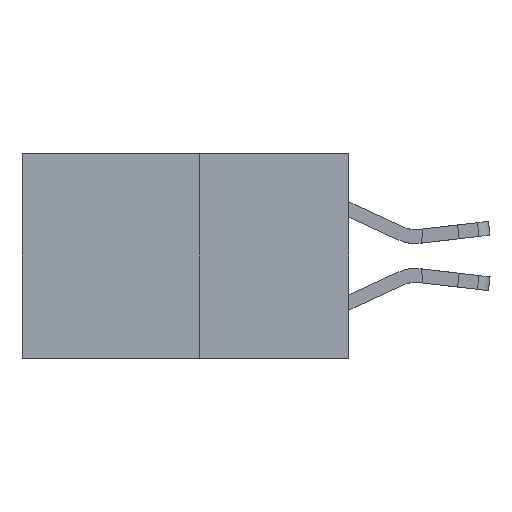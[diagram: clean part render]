
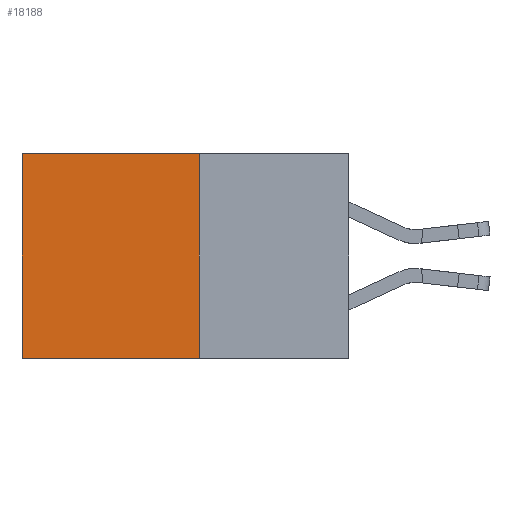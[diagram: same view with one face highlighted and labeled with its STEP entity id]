
A CAD part, left-side view. The second image highlights one B-rep face of the part: STEP entity #18188.
In plain terms, the highlighted planar face has unit normal (-1, 0, 0).
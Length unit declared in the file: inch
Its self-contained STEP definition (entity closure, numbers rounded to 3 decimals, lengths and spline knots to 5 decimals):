
#17 = VERTEX_POINT ( 'NONE', #15358 ) ;
#2304 = LINE ( 'NONE', #13840, #17884 ) ;
#2320 = CARTESIAN_POINT ( 'NONE',  ( 0.277, 0.59, -0.37 ) ) ;
#2510 = LINE ( 'NONE', #18720, #18080 ) ;
#2640 = CARTESIAN_POINT ( 'NONE',  ( 0.277, 0.27, -0.37 ) ) ;
#3442 = FACE_OUTER_BOUND ( 'NONE', #15813, .T. ) ;
#4179 = DIRECTION ( 'NONE',  ( 0., 0., -1. ) ) ;
#4262 = LINE ( 'NONE', #4757, #11395 ) ;
#4757 = CARTESIAN_POINT ( 'NONE',  ( 0.277, 0.27, -0.37 ) ) ;
#4841 = DIRECTION ( 'NONE',  ( 0., 1., 0. ) ) ;
#4848 = CARTESIAN_POINT ( 'NONE',  ( 0.277, 0.27, -0.37 ) ) ;
#5028 = EDGE_CURVE ( 'NONE', #17586, #14754, #2510, .T. ) ;
#5360 = CARTESIAN_POINT ( 'NONE',  ( 0.277, 0.27, 0. ) ) ;
#5529 = DIRECTION ( 'NONE',  ( 0., 1., 0. ) ) ;
#8305 = AXIS2_PLACEMENT_3D ( 'NONE', #2640, #13247, #4179 ) ;
#8691 = ORIENTED_EDGE ( 'NONE', *, *, #16693, .T. ) ;
#9034 = EDGE_CURVE ( 'NONE', #17586, #17, #17234, .T. ) ;
#9090 = EDGE_CURVE ( 'NONE', #14754, #9318, #4262, .T. ) ;
#9318 = VERTEX_POINT ( 'NONE', #2320 ) ;
#9626 = ORIENTED_EDGE ( 'NONE', *, *, #9090, .F. ) ;
#10334 = ORIENTED_EDGE ( 'NONE', *, *, #5028, .F. ) ;
#11395 = VECTOR ( 'NONE', #4841, 39.37008 ) ;
#11746 = PLANE ( 'NONE',  #8305 ) ;
#12327 = VECTOR ( 'NONE', #5529, 39.37008 ) ;
#12668 = CARTESIAN_POINT ( 'NONE',  ( 0.277, 0.27, 0. ) ) ;
#12875 = ORIENTED_EDGE ( 'NONE', *, *, #9034, .T. ) ;
#13247 = DIRECTION ( 'NONE',  ( 1., 0., 0. ) ) ;
#13840 = CARTESIAN_POINT ( 'NONE',  ( 0.277, 0.59, -0.37 ) ) ;
#14754 = VERTEX_POINT ( 'NONE', #4848 ) ;
#15352 = DIRECTION ( 'NONE',  ( 0., 0., -1. ) ) ;
#15358 = CARTESIAN_POINT ( 'NONE',  ( 0.277, 0.59, 0. ) ) ;
#15813 = EDGE_LOOP ( 'NONE', ( #8691, #9626, #10334, #12875 ) ) ;
#16693 = EDGE_CURVE ( 'NONE', #17, #9318, #2304, .T. ) ;
#17234 = LINE ( 'NONE', #5360, #12327 ) ;
#17586 = VERTEX_POINT ( 'NONE', #12668 ) ;
#17884 = VECTOR ( 'NONE', #15352, 39.37008 ) ;
#18080 = VECTOR ( 'NONE', #18573, 39.37008 ) ;
#18188 = ADVANCED_FACE ( 'NONE', ( #3442 ), #11746, .F. ) ;
#18573 = DIRECTION ( 'NONE',  ( 0., 0., -1. ) ) ;
#18720 = CARTESIAN_POINT ( 'NONE',  ( 0.277, 0.27, -0.37 ) ) ;
